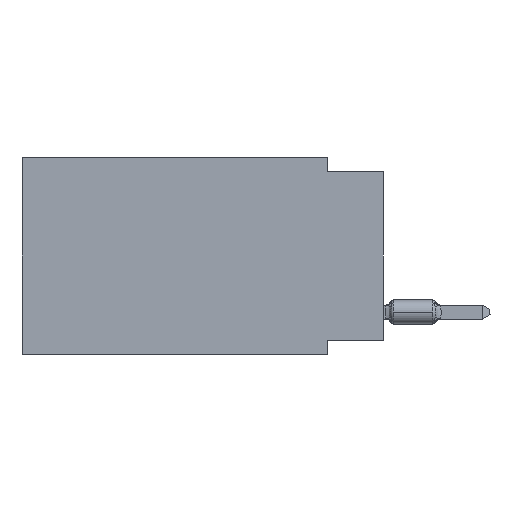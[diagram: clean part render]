
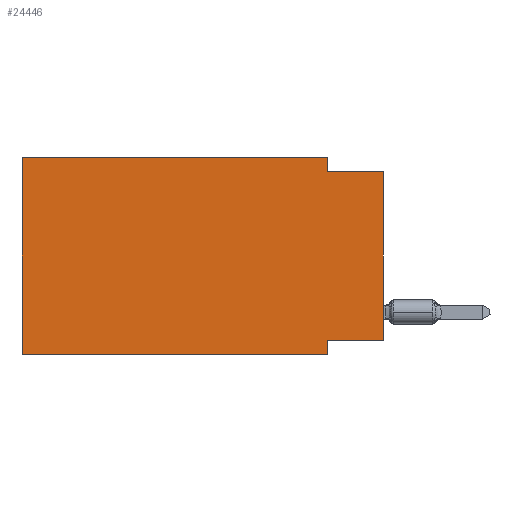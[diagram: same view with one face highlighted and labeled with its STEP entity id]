
A CAD part, left-side view. The second image highlights one B-rep face of the part: STEP entity #24446.
In plain terms, the highlighted planar face has unit normal (-1, 0, 0).
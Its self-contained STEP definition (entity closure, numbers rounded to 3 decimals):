
#215 = DIRECTION ( 'NONE',  ( 0., 0., 1. ) ) ;
#389 = EDGE_CURVE ( 'NONE', #5760, #26827, #2953, .T. ) ;
#641 = ORIENTED_EDGE ( 'NONE', *, *, #4754, .F. ) ;
#2722 = LINE ( 'NONE', #52877, #44333 ) ;
#2953 = LINE ( 'NONE', #6518, #11765 ) ;
#4173 = ORIENTED_EDGE ( 'NONE', *, *, #28256, .F. ) ;
#4203 = VERTEX_POINT ( 'NONE', #32680 ) ;
#4754 = EDGE_CURVE ( 'NONE', #4203, #18602, #25184, .T. ) ;
#5233 = LINE ( 'NONE', #37880, #17191 ) ;
#5730 = DIRECTION ( 'NONE',  ( 0., 0., -1. ) ) ;
#5760 = VERTEX_POINT ( 'NONE', #35918 ) ;
#6518 = CARTESIAN_POINT ( 'NONE',  ( 0., 2.54, -8.89 ) ) ;
#7710 = DIRECTION ( 'NONE',  ( 0., -1., 0. ) ) ;
#8704 = LINE ( 'NONE', #38573, #9789 ) ;
#9789 = VECTOR ( 'NONE', #215, 1000. ) ;
#9929 = DIRECTION ( 'NONE',  ( 0., 1., 0. ) ) ;
#10451 = CARTESIAN_POINT ( 'NONE',  ( 0., 16.383, -8.89 ) ) ;
#11765 = VECTOR ( 'NONE', #15280, 1000. ) ;
#13248 = EDGE_CURVE ( 'NONE', #17636, #5760, #34893, .T. ) ;
#13338 = CARTESIAN_POINT ( 'NONE',  ( 0., 0., -8.255 ) ) ;
#13598 = EDGE_CURVE ( 'NONE', #25141, #4203, #33201, .T. ) ;
#13979 = CARTESIAN_POINT ( 'NONE',  ( 0., 0., -0.635 ) ) ;
#14780 = DIRECTION ( 'NONE',  ( 1., 0., 0. ) ) ;
#15280 = DIRECTION ( 'NONE',  ( 0., 0., -1. ) ) ;
#15363 = AXIS2_PLACEMENT_3D ( 'NONE', #22737, #14780, #5730 ) ;
#15389 = VECTOR ( 'NONE', #7710, 1000. ) ;
#15659 = CARTESIAN_POINT ( 'NONE',  ( 0., 16.383, 0. ) ) ;
#16660 = CARTESIAN_POINT ( 'NONE',  ( 0., 2.54, -0.635 ) ) ;
#17191 = VECTOR ( 'NONE', #49946, 1000. ) ;
#17636 = VERTEX_POINT ( 'NONE', #13338 ) ;
#18602 = VERTEX_POINT ( 'NONE', #16660 ) ;
#19893 = VERTEX_POINT ( 'NONE', #10451 ) ;
#20740 = VECTOR ( 'NONE', #9929, 1000. ) ;
#22737 = CARTESIAN_POINT ( 'NONE',  ( 0., 16.383, 0. ) ) ;
#24446 = ADVANCED_FACE ( 'NONE', ( #43581 ), #39192, .F. ) ;
#25141 = VERTEX_POINT ( 'NONE', #50526 ) ;
#25184 = LINE ( 'NONE', #37801, #43997 ) ;
#25991 = DIRECTION ( 'NONE',  ( 0., 0., -1. ) ) ;
#26827 = VERTEX_POINT ( 'NONE', #33769 ) ;
#28256 = EDGE_CURVE ( 'NONE', #18602, #39631, #39726, .T. ) ;
#29468 = EDGE_CURVE ( 'NONE', #19893, #26827, #2722, .T. ) ;
#30762 = CARTESIAN_POINT ( 'NONE',  ( 0., 0., -8.255 ) ) ;
#31985 = VECTOR ( 'NONE', #47967, 1000. ) ;
#32680 = CARTESIAN_POINT ( 'NONE',  ( 0., 2.54, 0. ) ) ;
#33201 = LINE ( 'NONE', #15659, #15389 ) ;
#33769 = CARTESIAN_POINT ( 'NONE',  ( 0., 2.54, -8.89 ) ) ;
#34606 = CARTESIAN_POINT ( 'NONE',  ( 0., 0., -0.635 ) ) ;
#34893 = LINE ( 'NONE', #30762, #20740 ) ;
#35918 = CARTESIAN_POINT ( 'NONE',  ( 0., 2.54, -8.255 ) ) ;
#35997 = EDGE_LOOP ( 'NONE', ( #43516, #4173, #641, #38637, #41377, #41011, #39443, #37058 ) ) ;
#36189 = EDGE_CURVE ( 'NONE', #17636, #39631, #8704, .T. ) ;
#37058 = ORIENTED_EDGE ( 'NONE', *, *, #13248, .F. ) ;
#37801 = CARTESIAN_POINT ( 'NONE',  ( 0., 2.54, 0. ) ) ;
#37880 = CARTESIAN_POINT ( 'NONE',  ( 0., 16.383, 0. ) ) ;
#38573 = CARTESIAN_POINT ( 'NONE',  ( 0., 0., 0. ) ) ;
#38637 = ORIENTED_EDGE ( 'NONE', *, *, #13598, .F. ) ;
#39192 = PLANE ( 'NONE',  #15363 ) ;
#39443 = ORIENTED_EDGE ( 'NONE', *, *, #389, .F. ) ;
#39631 = VERTEX_POINT ( 'NONE', #34606 ) ;
#39726 = LINE ( 'NONE', #13979, #31985 ) ;
#41011 = ORIENTED_EDGE ( 'NONE', *, *, #29468, .T. ) ;
#41377 = ORIENTED_EDGE ( 'NONE', *, *, #45502, .F. ) ;
#43316 = DIRECTION ( 'NONE',  ( 0., -1., 0. ) ) ;
#43516 = ORIENTED_EDGE ( 'NONE', *, *, #36189, .T. ) ;
#43581 = FACE_OUTER_BOUND ( 'NONE', #35997, .T. ) ;
#43997 = VECTOR ( 'NONE', #25991, 1000. ) ;
#44333 = VECTOR ( 'NONE', #43316, 1000. ) ;
#45502 = EDGE_CURVE ( 'NONE', #19893, #25141, #5233, .T. ) ;
#47967 = DIRECTION ( 'NONE',  ( 0., -1., 0. ) ) ;
#49946 = DIRECTION ( 'NONE',  ( 0., 0., 1. ) ) ;
#50526 = CARTESIAN_POINT ( 'NONE',  ( 0., 16.383, 0. ) ) ;
#52877 = CARTESIAN_POINT ( 'NONE',  ( 0., 16.383, -8.89 ) ) ;
